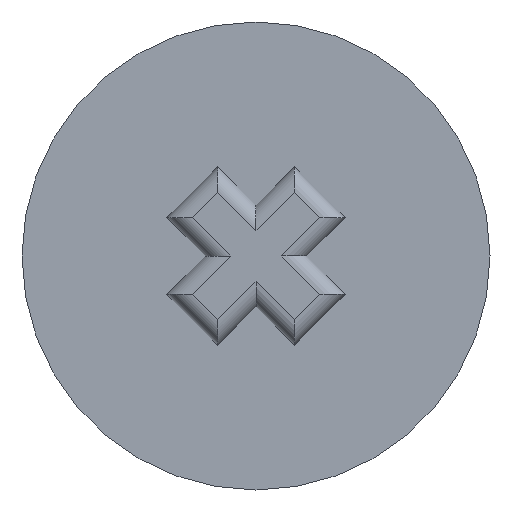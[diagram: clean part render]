
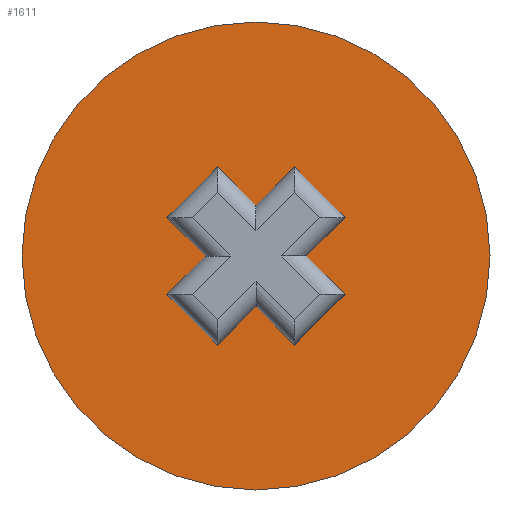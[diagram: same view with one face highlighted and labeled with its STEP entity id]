
A CAD part, left-side view. The second image highlights one B-rep face of the part: STEP entity #1611.
In plain terms, the highlighted planar face has unit normal (-1, 0, 0).
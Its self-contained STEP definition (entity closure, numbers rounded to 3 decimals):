
#7 = VERTEX_POINT ( 'NONE', #1517 ) ;
#33 = VERTEX_POINT ( 'NONE', #1539 ) ;
#63 = VERTEX_POINT ( 'NONE', #1564 ) ;
#65 = VERTEX_POINT ( 'NONE', #1566 ) ;
#128 = DIRECTION ( 'NONE',  ( 0., 0.707, -0.707 ) ) ;
#129 = DIRECTION ( 'NONE',  ( 0., -0.707, -0.707 ) ) ;
#131 = CARTESIAN_POINT ( 'NONE',  ( 0., 4.95, 2.121 ) ) ;
#141 = DIRECTION ( 'NONE',  ( 0., 0., -1. ) ) ;
#146 = DIRECTION ( 'NONE',  ( 1., 0., 0. ) ) ;
#149 = CARTESIAN_POINT ( 'NONE',  ( 0., 0., 0. ) ) ;
#157 = CARTESIAN_POINT ( 'NONE',  ( 0., 4.95, 2.121 ) ) ;
#180 = DIRECTION ( 'NONE',  ( 0., 0., -1. ) ) ;
#181 = DIRECTION ( 'NONE',  ( 1., 0., 0. ) ) ;
#191 = PLANE ( 'NONE',  #1766 ) ;
#197 = CARTESIAN_POINT ( 'NONE',  ( 0., 0., 0. ) ) ;
#292 = CARTESIAN_POINT ( 'NONE',  ( 0., -2.828, 0. ) ) ;
#297 = CARTESIAN_POINT ( 'NONE',  ( 0., 2.121, 4.95 ) ) ;
#301 = CARTESIAN_POINT ( 'NONE',  ( 0., 0., -2.828 ) ) ;
#304 = CARTESIAN_POINT ( 'NONE',  ( 0., -4.95, 2.121 ) ) ;
#307 = CARTESIAN_POINT ( 'NONE',  ( 0., 4.95, -2.121 ) ) ;
#310 = CARTESIAN_POINT ( 'NONE',  ( 0., 2.828, 0. ) ) ;
#313 = CARTESIAN_POINT ( 'NONE',  ( 0., 0., 2.828 ) ) ;
#316 = CARTESIAN_POINT ( 'NONE',  ( 0., 2.121, -4.95 ) ) ;
#318 = CARTESIAN_POINT ( 'NONE',  ( 0., -2.121, -4.95 ) ) ;
#353 = DIRECTION ( 'NONE',  ( 0., 0.707, 0.707 ) ) ;
#366 = CARTESIAN_POINT ( 'NONE',  ( 0., 2.121, 4.95 ) ) ;
#413 = CARTESIAN_POINT ( 'NONE',  ( 0., 0., 0. ) ) ;
#414 = DIRECTION ( 'NONE',  ( 1., 0., 0. ) ) ;
#415 = DIRECTION ( 'NONE',  ( 0., 0., -1. ) ) ;
#416 = CARTESIAN_POINT ( 'NONE',  ( 0., -2.121, 4.95 ) ) ;
#417 = DIRECTION ( 'NONE',  ( 0., 0.707, -0.707 ) ) ;
#418 = CARTESIAN_POINT ( 'NONE',  ( 0., -4.95, 2.121 ) ) ;
#419 = DIRECTION ( 'NONE',  ( 0., 0.707, 0.707 ) ) ;
#420 = CARTESIAN_POINT ( 'NONE',  ( 0., -4.95, 2.121 ) ) ;
#421 = DIRECTION ( 'NONE',  ( 0., -0.707, 0.707 ) ) ;
#422 = CARTESIAN_POINT ( 'NONE',  ( 0., 2.121, 4.95 ) ) ;
#423 = DIRECTION ( 'NONE',  ( 0., 0.707, 0.707 ) ) ;
#424 = CARTESIAN_POINT ( 'NONE',  ( 0., -2.121, -4.95 ) ) ;
#425 = DIRECTION ( 'NONE',  ( 0., -0.707, 0.707 ) ) ;
#426 = CARTESIAN_POINT ( 'NONE',  ( 0., 4.95, 2.121 ) ) ;
#427 = DIRECTION ( 'NONE',  ( 0., -0.707, -0.707 ) ) ;
#428 = CARTESIAN_POINT ( 'NONE',  ( 0., -4.95, 2.121 ) ) ;
#429 = DIRECTION ( 'NONE',  ( 0., -0.707, 0.707 ) ) ;
#430 = CARTESIAN_POINT ( 'NONE',  ( 0., 2.121, -4.95 ) ) ;
#431 = DIRECTION ( 'NONE',  ( 0., -0.707, -0.707 ) ) ;
#432 = CARTESIAN_POINT ( 'NONE',  ( 0., -2.121, 4.95 ) ) ;
#433 = DIRECTION ( 'NONE',  ( 0., 0.707, -0.707 ) ) ;
#572 = CIRCLE ( 'NONE', #1821, 13. ) ;
#574 = LINE ( 'NONE', #366, #576 ) ;
#575 = LINE ( 'NONE', #416, #578 ) ;
#576 = VECTOR ( 'NONE', #353, 1000. ) ;
#577 = LINE ( 'NONE', #418, #580 ) ;
#578 = VECTOR ( 'NONE', #417, 1000. ) ;
#579 = LINE ( 'NONE', #420, #582 ) ;
#580 = VECTOR ( 'NONE', #419, 1000. ) ;
#581 = LINE ( 'NONE', #422, #584 ) ;
#582 = VECTOR ( 'NONE', #421, 1000. ) ;
#583 = LINE ( 'NONE', #424, #586 ) ;
#584 = VECTOR ( 'NONE', #423, 1000. ) ;
#585 = LINE ( 'NONE', #426, #588 ) ;
#586 = VECTOR ( 'NONE', #425, 1000. ) ;
#587 = LINE ( 'NONE', #428, #590 ) ;
#588 = VECTOR ( 'NONE', #427, 1000. ) ;
#589 = LINE ( 'NONE', #430, #592 ) ;
#590 = VECTOR ( 'NONE', #429, 1000. ) ;
#591 = LINE ( 'NONE', #432, #594 ) ;
#592 = VECTOR ( 'NONE', #431, 1000. ) ;
#594 = VECTOR ( 'NONE', #433, 1000. ) ;
#855 = VERTEX_POINT ( 'NONE', #1574 ) ;
#972 = CIRCLE ( 'NONE', #1748, 13. ) ;
#980 = LINE ( 'NONE', #157, #987 ) ;
#982 = LINE ( 'NONE', #131, #985 ) ;
#985 = VECTOR ( 'NONE', #129, 1000. ) ;
#987 = VECTOR ( 'NONE', #128, 1000. ) ;
#1073 = FACE_OUTER_BOUND ( 'NONE', #1417, .T. ) ;
#1076 = FACE_BOUND ( 'NONE', #1433, .T. ) ;
#1247 = ORIENTED_EDGE ( 'NONE', *, *, #1737, .F. ) ;
#1248 = ORIENTED_EDGE ( 'NONE', *, *, #1469, .F. ) ;
#1249 = ORIENTED_EDGE ( 'NONE', *, *, #1738, .F. ) ;
#1250 = ORIENTED_EDGE ( 'NONE', *, *, #1739, .F. ) ;
#1251 = ORIENTED_EDGE ( 'NONE', *, *, #1740, .F. ) ;
#1252 = ORIENTED_EDGE ( 'NONE', *, *, #1741, .F. ) ;
#1253 = ORIENTED_EDGE ( 'NONE', *, *, #1742, .F. ) ;
#1254 = ORIENTED_EDGE ( 'NONE', *, *, #1743, .F. ) ;
#1255 = ORIENTED_EDGE ( 'NONE', *, *, #1744, .F. ) ;
#1256 = ORIENTED_EDGE ( 'NONE', *, *, #1745, .F. ) ;
#1257 = ORIENTED_EDGE ( 'NONE', *, *, #1746, .F. ) ;
#1258 = ORIENTED_EDGE ( 'NONE', *, *, #1747, .F. ) ;
#1259 = ORIENTED_EDGE ( 'NONE', *, *, #1474, .F. ) ;
#1260 = ORIENTED_EDGE ( 'NONE', *, *, #1475, .F. ) ;
#1417 = EDGE_LOOP ( 'NONE', ( #1247, #1248 ) ) ;
#1433 = EDGE_LOOP ( 'NONE', ( #1249, #1250, #1251, #1252, #1253, #1254, #1255, #1256, #1257, #1258, #1259, #1260 ) ) ;
#1439 = VERTEX_POINT ( 'NONE', #310 ) ;
#1440 = VERTEX_POINT ( 'NONE', #307 ) ;
#1445 = VERTEX_POINT ( 'NONE', #304 ) ;
#1446 = VERTEX_POINT ( 'NONE', #318 ) ;
#1447 = VERTEX_POINT ( 'NONE', #301 ) ;
#1448 = VERTEX_POINT ( 'NONE', #316 ) ;
#1449 = VERTEX_POINT ( 'NONE', #297 ) ;
#1450 = VERTEX_POINT ( 'NONE', #313 ) ;
#1451 = VERTEX_POINT ( 'NONE', #292 ) ;
#1469 = EDGE_CURVE ( 'NONE', #7, #33, #972, .T. ) ;
#1474 = EDGE_CURVE ( 'NONE', #855, #1439, #982, .T. ) ;
#1475 = EDGE_CURVE ( 'NONE', #1449, #855, #980, .T. ) ;
#1517 = CARTESIAN_POINT ( 'NONE',  ( 0., 0., -13. ) ) ;
#1539 = CARTESIAN_POINT ( 'NONE',  ( 0., 0., 13. ) ) ;
#1564 = CARTESIAN_POINT ( 'NONE',  ( 0., -4.95, -2.121 ) ) ;
#1566 = CARTESIAN_POINT ( 'NONE',  ( 0., -2.121, 4.95 ) ) ;
#1574 = CARTESIAN_POINT ( 'NONE',  ( 0., 4.95, 2.121 ) ) ;
#1611 = ADVANCED_FACE ( 'NONE', ( #1073, #1076 ), #191, .F. ) ;
#1737 = EDGE_CURVE ( 'NONE', #33, #7, #572, .T. ) ;
#1738 = EDGE_CURVE ( 'NONE', #1450, #1449, #574, .T. ) ;
#1739 = EDGE_CURVE ( 'NONE', #65, #1450, #575, .T. ) ;
#1740 = EDGE_CURVE ( 'NONE', #1445, #65, #577, .T. ) ;
#1741 = EDGE_CURVE ( 'NONE', #1451, #1445, #579, .T. ) ;
#1742 = EDGE_CURVE ( 'NONE', #63, #1451, #581, .T. ) ;
#1743 = EDGE_CURVE ( 'NONE', #1446, #63, #583, .T. ) ;
#1744 = EDGE_CURVE ( 'NONE', #1447, #1446, #585, .T. ) ;
#1745 = EDGE_CURVE ( 'NONE', #1448, #1447, #587, .T. ) ;
#1746 = EDGE_CURVE ( 'NONE', #1440, #1448, #589, .T. ) ;
#1747 = EDGE_CURVE ( 'NONE', #1439, #1440, #591, .T. ) ;
#1748 = AXIS2_PLACEMENT_3D ( 'NONE', #149, #146, #141 ) ;
#1766 = AXIS2_PLACEMENT_3D ( 'NONE', #197, #181, #180 ) ;
#1821 = AXIS2_PLACEMENT_3D ( 'NONE', #413, #414, #415 ) ;
